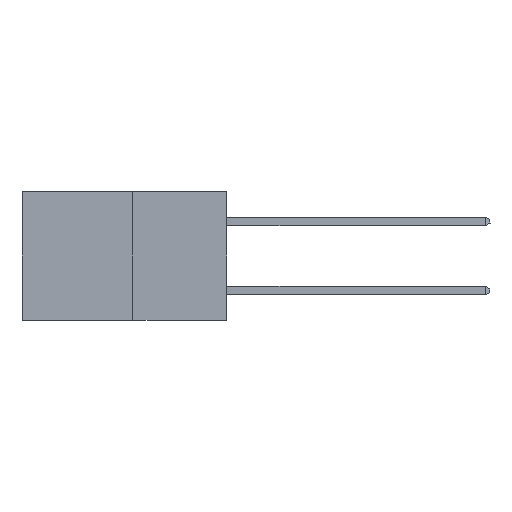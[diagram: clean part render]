
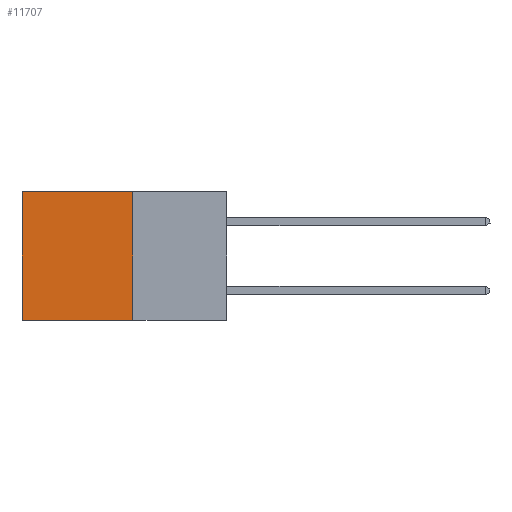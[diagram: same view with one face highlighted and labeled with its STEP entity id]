
A CAD part, left-side view. The second image highlights one B-rep face of the part: STEP entity #11707.
In plain terms, the highlighted planar face has unit normal (-1, 0, 0).
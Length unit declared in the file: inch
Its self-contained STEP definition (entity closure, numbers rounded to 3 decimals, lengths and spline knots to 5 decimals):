
#186 = DIRECTION ( 'NONE',  ( 0., 0., -1. ) ) ;
#381 = VECTOR ( 'NONE', #4398, 39.37008 ) ;
#389 = ORIENTED_EDGE ( 'NONE', *, *, #6179, .T. ) ;
#412 = DIRECTION ( 'NONE',  ( 0., 1., 0. ) ) ;
#461 = CARTESIAN_POINT ( 'NONE',  ( 0.277, 0.27, 0. ) ) ;
#485 = CARTESIAN_POINT ( 'NONE',  ( 0.277, 0.59, 0. ) ) ;
#698 = LINE ( 'NONE', #11836, #381 ) ;
#723 = VERTEX_POINT ( 'NONE', #7498 ) ;
#922 = PLANE ( 'NONE',  #4468 ) ;
#1082 = VERTEX_POINT ( 'NONE', #9520 ) ;
#2511 = CARTESIAN_POINT ( 'NONE',  ( 0.277, 0.27, -0.37 ) ) ;
#2545 = LINE ( 'NONE', #2511, #9745 ) ;
#2792 = EDGE_CURVE ( 'NONE', #4516, #723, #698, .T. ) ;
#2831 = EDGE_LOOP ( 'NONE', ( #5012, #9195, #9087, #389 ) ) ;
#3004 = DIRECTION ( 'NONE',  ( 0., 0., -1. ) ) ;
#3245 = EDGE_CURVE ( 'NONE', #5130, #723, #10135, .T. ) ;
#3632 = EDGE_CURVE ( 'NONE', #1082, #4516, #2545, .T. ) ;
#4398 = DIRECTION ( 'NONE',  ( 0., 1., 0. ) ) ;
#4468 = AXIS2_PLACEMENT_3D ( 'NONE', #5888, #9504, #3004 ) ;
#4516 = VERTEX_POINT ( 'NONE', #11700 ) ;
#4624 = VECTOR ( 'NONE', #412, 39.37008 ) ;
#5012 = ORIENTED_EDGE ( 'NONE', *, *, #3245, .T. ) ;
#5130 = VERTEX_POINT ( 'NONE', #485 ) ;
#5357 = VECTOR ( 'NONE', #186, 39.37008 ) ;
#5888 = CARTESIAN_POINT ( 'NONE',  ( 0.277, 0.27, -0.37 ) ) ;
#6179 = EDGE_CURVE ( 'NONE', #1082, #5130, #6895, .T. ) ;
#6718 = CARTESIAN_POINT ( 'NONE',  ( 0.277, 0.59, -0.37 ) ) ;
#6895 = LINE ( 'NONE', #461, #4624 ) ;
#7498 = CARTESIAN_POINT ( 'NONE',  ( 0.277, 0.59, -0.37 ) ) ;
#9087 = ORIENTED_EDGE ( 'NONE', *, *, #3632, .F. ) ;
#9195 = ORIENTED_EDGE ( 'NONE', *, *, #2792, .F. ) ;
#9469 = DIRECTION ( 'NONE',  ( 0., 0., -1. ) ) ;
#9504 = DIRECTION ( 'NONE',  ( 1., 0., 0. ) ) ;
#9520 = CARTESIAN_POINT ( 'NONE',  ( 0.277, 0.27, 0. ) ) ;
#9745 = VECTOR ( 'NONE', #9469, 39.37008 ) ;
#10135 = LINE ( 'NONE', #6718, #5357 ) ;
#11641 = FACE_OUTER_BOUND ( 'NONE', #2831, .T. ) ;
#11700 = CARTESIAN_POINT ( 'NONE',  ( 0.277, 0.27, -0.37 ) ) ;
#11707 = ADVANCED_FACE ( 'NONE', ( #11641 ), #922, .F. ) ;
#11836 = CARTESIAN_POINT ( 'NONE',  ( 0.277, 0.27, -0.37 ) ) ;
